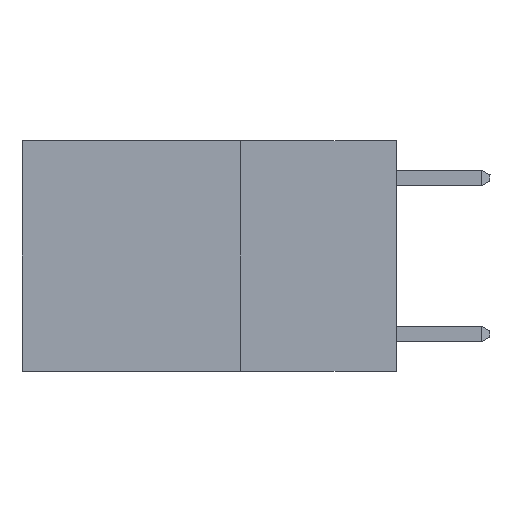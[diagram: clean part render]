
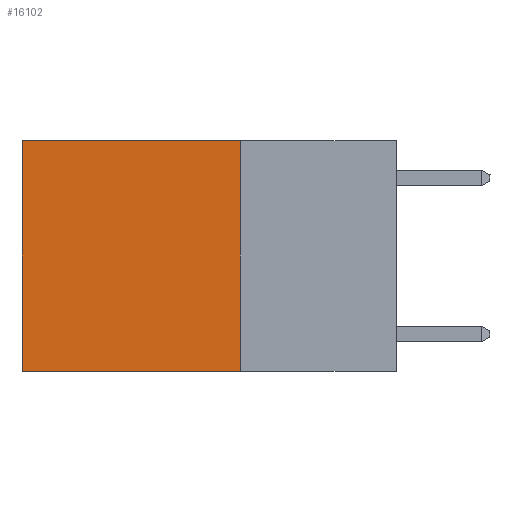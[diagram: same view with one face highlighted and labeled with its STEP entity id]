
A CAD part, left-side view. The second image highlights one B-rep face of the part: STEP entity #16102.
In plain terms, the highlighted planar face has unit normal (-1, 0, 0).
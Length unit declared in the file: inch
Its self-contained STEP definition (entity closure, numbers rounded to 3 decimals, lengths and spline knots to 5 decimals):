
#238 = PLANE ( 'NONE',  #16085 ) ;
#386 = CARTESIAN_POINT ( 'NONE',  ( 0.2625, 0.6, -0.37 ) ) ;
#437 = VERTEX_POINT ( 'NONE', #1949 ) ;
#1327 = DIRECTION ( 'NONE',  ( 0., 0., -1. ) ) ;
#1949 = CARTESIAN_POINT ( 'NONE',  ( 0.2625, 0.6, 0. ) ) ;
#2579 = CARTESIAN_POINT ( 'NONE',  ( 0.2625, 0.25, -0.37 ) ) ;
#3302 = EDGE_CURVE ( 'NONE', #14802, #437, #12297, .T. ) ;
#3691 = EDGE_CURVE ( 'NONE', #12685, #4357, #8232, .T. ) ;
#4048 = LINE ( 'NONE', #15091, #8076 ) ;
#4166 = VECTOR ( 'NONE', #5553, 39.37008 ) ;
#4357 = VERTEX_POINT ( 'NONE', #386 ) ;
#4483 = VECTOR ( 'NONE', #8166, 39.37008 ) ;
#5553 = DIRECTION ( 'NONE',  ( 0., 1., 0. ) ) ;
#5658 = FACE_OUTER_BOUND ( 'NONE', #17372, .T. ) ;
#6613 = CARTESIAN_POINT ( 'NONE',  ( 0.2625, 0.25, 0. ) ) ;
#7917 = LINE ( 'NONE', #13405, #16563 ) ;
#8076 = VECTOR ( 'NONE', #1327, 39.37008 ) ;
#8166 = DIRECTION ( 'NONE',  ( 0., 1., 0. ) ) ;
#8232 = LINE ( 'NONE', #2579, #4166 ) ;
#9559 = EDGE_CURVE ( 'NONE', #437, #4357, #4048, .T. ) ;
#9811 = ORIENTED_EDGE ( 'NONE', *, *, #9559, .T. ) ;
#10715 = DIRECTION ( 'NONE',  ( 0., 0., -1. ) ) ;
#10939 = ORIENTED_EDGE ( 'NONE', *, *, #3302, .T. ) ;
#12297 = LINE ( 'NONE', #16265, #4483 ) ;
#12474 = DIRECTION ( 'NONE',  ( 1., 0., 0. ) ) ;
#12604 = EDGE_CURVE ( 'NONE', #14802, #12685, #7917, .T. ) ;
#12685 = VERTEX_POINT ( 'NONE', #13846 ) ;
#13405 = CARTESIAN_POINT ( 'NONE',  ( 0.2625, 0.25, 0. ) ) ;
#13651 = CARTESIAN_POINT ( 'NONE',  ( 0.2625, 0.25, 0. ) ) ;
#13846 = CARTESIAN_POINT ( 'NONE',  ( 0.2625, 0.25, -0.37 ) ) ;
#14590 = ORIENTED_EDGE ( 'NONE', *, *, #3691, .F. ) ;
#14802 = VERTEX_POINT ( 'NONE', #6613 ) ;
#15004 = DIRECTION ( 'NONE',  ( 0., 0., -1. ) ) ;
#15091 = CARTESIAN_POINT ( 'NONE',  ( 0.2625, 0.6, 0. ) ) ;
#15628 = ORIENTED_EDGE ( 'NONE', *, *, #12604, .F. ) ;
#16085 = AXIS2_PLACEMENT_3D ( 'NONE', #13651, #12474, #15004 ) ;
#16102 = ADVANCED_FACE ( 'NONE', ( #5658 ), #238, .F. ) ;
#16265 = CARTESIAN_POINT ( 'NONE',  ( 0.2625, 0.25, 0. ) ) ;
#16563 = VECTOR ( 'NONE', #10715, 39.37008 ) ;
#17372 = EDGE_LOOP ( 'NONE', ( #9811, #14590, #15628, #10939 ) ) ;
